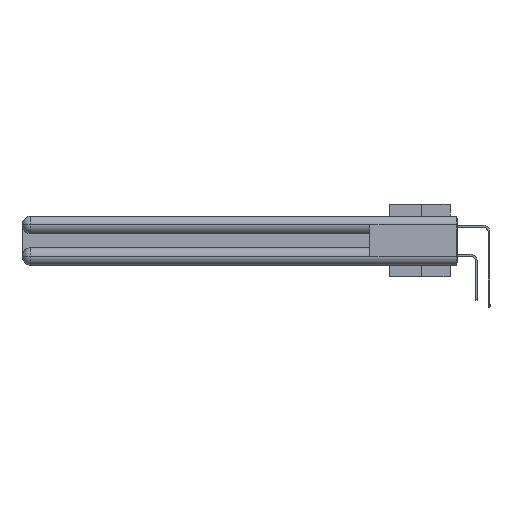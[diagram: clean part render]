
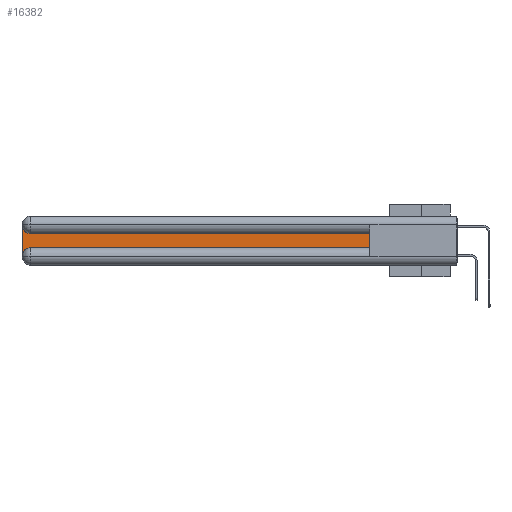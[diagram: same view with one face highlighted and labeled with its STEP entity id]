
A CAD part, left-side view. The second image highlights one B-rep face of the part: STEP entity #16382.
In plain terms, the highlighted planar face has unit normal (-1, 0, 0).
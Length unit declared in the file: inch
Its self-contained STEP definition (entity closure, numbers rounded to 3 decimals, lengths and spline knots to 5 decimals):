
#831 = EDGE_CURVE ( 'NONE', #14907, #967, #35627, .T. ) ;
#967 = VERTEX_POINT ( 'NONE', #11309 ) ;
#1930 = ORIENTED_EDGE ( 'NONE', *, *, #35935, .T. ) ;
#3912 = CARTESIAN_POINT ( 'NONE',  ( 0.075, 0.6, -0.2175 ) ) ;
#4752 = VECTOR ( 'NONE', #30667, 39.37008 ) ;
#5040 = DIRECTION ( 'NONE',  ( 0., 0., -1. ) ) ;
#5240 = EDGE_CURVE ( 'NONE', #27819, #11907, #5326, .T. ) ;
#5326 = LINE ( 'NONE', #26979, #4752 ) ;
#5344 = LINE ( 'NONE', #39553, #11464 ) ;
#5760 = CARTESIAN_POINT ( 'NONE',  ( 0.075, 2.94, -0.2175 ) ) ;
#5811 = ORIENTED_EDGE ( 'NONE', *, *, #5240, .T. ) ;
#6411 = EDGE_CURVE ( 'NONE', #10585, #14907, #7090, .T. ) ;
#6650 = DIRECTION ( 'NONE',  ( 0., 0., -1. ) ) ;
#7090 = CIRCLE ( 'NONE', #22914, 0.06 ) ;
#7485 = CARTESIAN_POINT ( 'NONE',  ( 0.075, 2.94, -0.1225 ) ) ;
#8113 = ORIENTED_EDGE ( 'NONE', *, *, #6411, .T. ) ;
#8122 = CARTESIAN_POINT ( 'NONE',  ( 0.075, 3., -0.2175 ) ) ;
#8337 = LINE ( 'NONE', #8122, #35734 ) ;
#10112 = PLANE ( 'NONE',  #22229 ) ;
#10585 = VERTEX_POINT ( 'NONE', #33709 ) ;
#11309 = CARTESIAN_POINT ( 'NONE',  ( 0.075, 0.6, -0.2175 ) ) ;
#11464 = VECTOR ( 'NONE', #17923, 39.37008 ) ;
#11907 = VERTEX_POINT ( 'NONE', #7485 ) ;
#11988 = VECTOR ( 'NONE', #28632, 39.37008 ) ;
#13869 = CARTESIAN_POINT ( 'NONE',  ( 0.075, 2.94, -0.2775 ) ) ;
#14907 = VERTEX_POINT ( 'NONE', #5760 ) ;
#16382 = ADVANCED_FACE ( 'NONE', ( #25782 ), #10112, .F. ) ;
#16902 = DIRECTION ( 'NONE',  ( 0., 0., -1. ) ) ;
#17923 = DIRECTION ( 'NONE',  ( 0., 0., 1. ) ) ;
#19764 = CARTESIAN_POINT ( 'NONE',  ( 0.075, 0.6, -0.1225 ) ) ;
#20010 = DIRECTION ( 'NONE',  ( 1., 0., 0. ) ) ;
#21919 = AXIS2_PLACEMENT_3D ( 'NONE', #37625, #28358, #40529 ) ;
#22229 = AXIS2_PLACEMENT_3D ( 'NONE', #22281, #20010, #16902 ) ;
#22281 = CARTESIAN_POINT ( 'NONE',  ( 0.075, 3., -0.1225 ) ) ;
#22668 = EDGE_CURVE ( 'NONE', #23028, #10585, #8337, .T. ) ;
#22914 = AXIS2_PLACEMENT_3D ( 'NONE', #13869, #29111, #6650 ) ;
#23028 = VERTEX_POINT ( 'NONE', #36309 ) ;
#24259 = EDGE_CURVE ( 'NONE', #967, #27819, #5344, .T. ) ;
#25782 = FACE_OUTER_BOUND ( 'NONE', #36375, .T. ) ;
#25861 = CIRCLE ( 'NONE', #21919, 0.06 ) ;
#26475 = ORIENTED_EDGE ( 'NONE', *, *, #22668, .T. ) ;
#26839 = ORIENTED_EDGE ( 'NONE', *, *, #24259, .T. ) ;
#26979 = CARTESIAN_POINT ( 'NONE',  ( 0.075, 0.6, -0.1225 ) ) ;
#27819 = VERTEX_POINT ( 'NONE', #19764 ) ;
#28358 = DIRECTION ( 'NONE',  ( 1., 0., 0. ) ) ;
#28632 = DIRECTION ( 'NONE',  ( 0., -1., 0. ) ) ;
#29111 = DIRECTION ( 'NONE',  ( 1., 0., 0. ) ) ;
#30667 = DIRECTION ( 'NONE',  ( 0., 1., 0. ) ) ;
#33232 = ORIENTED_EDGE ( 'NONE', *, *, #831, .T. ) ;
#33709 = CARTESIAN_POINT ( 'NONE',  ( 0.075, 3., -0.2775 ) ) ;
#35627 = LINE ( 'NONE', #3912, #11988 ) ;
#35734 = VECTOR ( 'NONE', #5040, 39.37008 ) ;
#35935 = EDGE_CURVE ( 'NONE', #11907, #23028, #25861, .T. ) ;
#36309 = CARTESIAN_POINT ( 'NONE',  ( 0.075, 3., -0.0625 ) ) ;
#36375 = EDGE_LOOP ( 'NONE', ( #5811, #1930, #26475, #8113, #33232, #26839 ) ) ;
#37625 = CARTESIAN_POINT ( 'NONE',  ( 0.075, 2.94, -0.0625 ) ) ;
#39553 = CARTESIAN_POINT ( 'NONE',  ( 0.075, 0.6, -0.2175 ) ) ;
#40529 = DIRECTION ( 'NONE',  ( 0., 0., -1. ) ) ;
